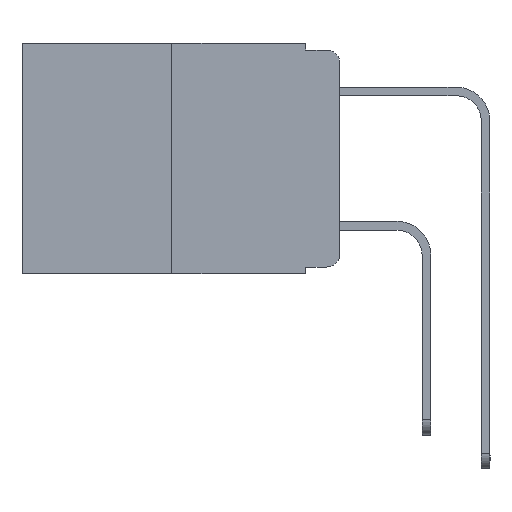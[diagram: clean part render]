
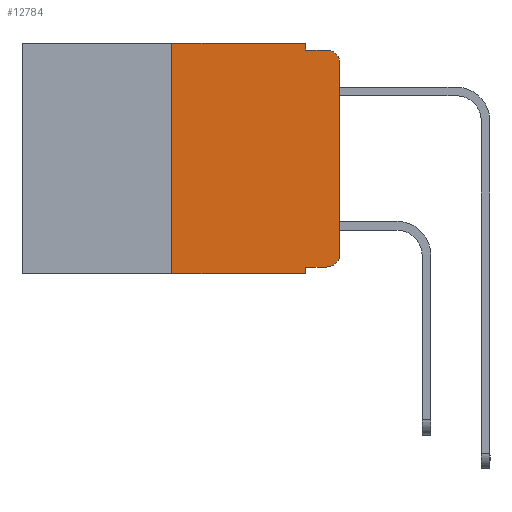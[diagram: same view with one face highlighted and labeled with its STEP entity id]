
A CAD part, left-side view. The second image highlights one B-rep face of the part: STEP entity #12784.
In plain terms, the highlighted planar face has unit normal (-1, 0, 0).
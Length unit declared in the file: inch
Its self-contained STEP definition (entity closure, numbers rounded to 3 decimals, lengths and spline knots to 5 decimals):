
#77 = CARTESIAN_POINT ( 'NONE',  ( 0., 0.051, 0. ) ) ;
#140 = DIRECTION ( 'NONE',  ( 0., 0., -1. ) ) ;
#180 = DIRECTION ( 'NONE',  ( 0., 0., 1. ) ) ;
#378 = VECTOR ( 'NONE', #5971, 39.37008 ) ;
#610 = CARTESIAN_POINT ( 'NONE',  ( 0., 0.051, -0.01 ) ) ;
#616 = LINE ( 'NONE', #4800, #12299 ) ;
#624 = DIRECTION ( 'NONE',  ( 0., -1., 0. ) ) ;
#729 = VERTEX_POINT ( 'NONE', #12332 ) ;
#802 = VECTOR ( 'NONE', #822, 39.37008 ) ;
#822 = DIRECTION ( 'NONE',  ( 0., -1., 0. ) ) ;
#1186 = ORIENTED_EDGE ( 'NONE', *, *, #3852, .T. ) ;
#1196 = ORIENTED_EDGE ( 'NONE', *, *, #6794, .F. ) ;
#1293 = FACE_OUTER_BOUND ( 'NONE', #4846, .T. ) ;
#1451 = ORIENTED_EDGE ( 'NONE', *, *, #1779, .F. ) ;
#1779 = EDGE_CURVE ( 'NONE', #729, #6059, #11518, .T. ) ;
#1817 = ORIENTED_EDGE ( 'NONE', *, *, #9703, .F. ) ;
#1902 = EDGE_CURVE ( 'NONE', #5700, #4947, #2800, .T. ) ;
#2146 = LINE ( 'NONE', #12782, #4140 ) ;
#2340 = DIRECTION ( 'NONE',  ( 0., 0., 1. ) ) ;
#2369 = ORIENTED_EDGE ( 'NONE', *, *, #7929, .T. ) ;
#2800 = CIRCLE ( 'NONE', #13323, 0.02 ) ;
#2854 = CARTESIAN_POINT ( 'NONE',  ( 0., 0.02, -0.333 ) ) ;
#2870 = LINE ( 'NONE', #9394, #802 ) ;
#3072 = CARTESIAN_POINT ( 'NONE',  ( 0., 0.25, -0.343 ) ) ;
#3339 = DIRECTION ( 'NONE',  ( 1., 0., 0. ) ) ;
#3549 = CARTESIAN_POINT ( 'NONE',  ( 0., 0.473, 0. ) ) ;
#3610 = VERTEX_POINT ( 'NONE', #5218 ) ;
#3654 = VECTOR ( 'NONE', #8582, 39.37008 ) ;
#3680 = CARTESIAN_POINT ( 'NONE',  ( 0., 0.051, -0.01 ) ) ;
#3817 = LINE ( 'NONE', #3680, #378 ) ;
#3852 = EDGE_CURVE ( 'NONE', #11744, #11363, #11862, .T. ) ;
#3890 = EDGE_CURVE ( 'NONE', #12164, #11363, #616, .T. ) ;
#4140 = VECTOR ( 'NONE', #2340, 39.37008 ) ;
#4532 = EDGE_CURVE ( 'NONE', #11744, #13049, #2146, .T. ) ;
#4800 = CARTESIAN_POINT ( 'NONE',  ( 0., 0.051, 0. ) ) ;
#4807 = CARTESIAN_POINT ( 'NONE',  ( 0., 0.02, -0.03 ) ) ;
#4846 = EDGE_LOOP ( 'NONE', ( #7281, #13448, #1817, #1451, #1196, #11756, #1186, #13243, #2369, #10557 ) ) ;
#4947 = VERTEX_POINT ( 'NONE', #11326 ) ;
#5218 = CARTESIAN_POINT ( 'NONE',  ( 0., 0., -0.03 ) ) ;
#5402 = CARTESIAN_POINT ( 'NONE',  ( 0., 0., 0. ) ) ;
#5700 = VERTEX_POINT ( 'NONE', #2854 ) ;
#5971 = DIRECTION ( 'NONE',  ( 0., -1., 0. ) ) ;
#6059 = VERTEX_POINT ( 'NONE', #610 ) ;
#6112 = AXIS2_PLACEMENT_3D ( 'NONE', #4807, #13035, #7919 ) ;
#6231 = CARTESIAN_POINT ( 'NONE',  ( 0., 0.051, -0.333 ) ) ;
#6718 = DIRECTION ( 'NONE',  ( -1., 0., 0. ) ) ;
#6727 = CARTESIAN_POINT ( 'NONE',  ( 0., 0.473, -0.343 ) ) ;
#6794 = EDGE_CURVE ( 'NONE', #13049, #729, #2870, .T. ) ;
#6804 = LINE ( 'NONE', #10985, #8304 ) ;
#6867 = DIRECTION ( 'NONE',  ( 0., 0., -1. ) ) ;
#7281 = ORIENTED_EDGE ( 'NONE', *, *, #10033, .T. ) ;
#7380 = VERTEX_POINT ( 'NONE', #11757 ) ;
#7833 = CARTESIAN_POINT ( 'NONE',  ( 0., 0.02, -0.313 ) ) ;
#7866 = CIRCLE ( 'NONE', #6112, 0.02 ) ;
#7919 = DIRECTION ( 'NONE',  ( 0., 0., -1. ) ) ;
#7929 = EDGE_CURVE ( 'NONE', #12164, #5700, #6804, .T. ) ;
#7941 = EDGE_CURVE ( 'NONE', #3610, #7380, #7866, .T. ) ;
#8304 = VECTOR ( 'NONE', #624, 39.37008 ) ;
#8497 = LINE ( 'NONE', #5402, #11776 ) ;
#8582 = DIRECTION ( 'NONE',  ( 0., 0., -1. ) ) ;
#9394 = CARTESIAN_POINT ( 'NONE',  ( 0., 0.473, 0. ) ) ;
#9446 = AXIS2_PLACEMENT_3D ( 'NONE', #3549, #3339, #140 ) ;
#9470 = CARTESIAN_POINT ( 'NONE',  ( 0., 0.051, -0.343 ) ) ;
#9703 = EDGE_CURVE ( 'NONE', #6059, #7380, #3817, .T. ) ;
#10033 = EDGE_CURVE ( 'NONE', #4947, #3610, #8497, .T. ) ;
#10557 = ORIENTED_EDGE ( 'NONE', *, *, #1902, .T. ) ;
#10908 = DIRECTION ( 'NONE',  ( 0., -1., 0. ) ) ;
#10983 = VECTOR ( 'NONE', #10908, 39.37008 ) ;
#10985 = CARTESIAN_POINT ( 'NONE',  ( 0., 0.051, -0.333 ) ) ;
#11326 = CARTESIAN_POINT ( 'NONE',  ( 0., 0., -0.313 ) ) ;
#11363 = VERTEX_POINT ( 'NONE', #9470 ) ;
#11380 = CARTESIAN_POINT ( 'NONE',  ( 0., 0.25, 0. ) ) ;
#11518 = LINE ( 'NONE', #77, #3654 ) ;
#11744 = VERTEX_POINT ( 'NONE', #3072 ) ;
#11756 = ORIENTED_EDGE ( 'NONE', *, *, #4532, .F. ) ;
#11757 = CARTESIAN_POINT ( 'NONE',  ( 0., 0.02, -0.01 ) ) ;
#11776 = VECTOR ( 'NONE', #180, 39.37008 ) ;
#11862 = LINE ( 'NONE', #6727, #10983 ) ;
#11926 = PLANE ( 'NONE',  #9446 ) ;
#12057 = DIRECTION ( 'NONE',  ( 0., 0., -1. ) ) ;
#12164 = VERTEX_POINT ( 'NONE', #6231 ) ;
#12299 = VECTOR ( 'NONE', #6867, 39.37008 ) ;
#12332 = CARTESIAN_POINT ( 'NONE',  ( 0., 0.051, 0. ) ) ;
#12782 = CARTESIAN_POINT ( 'NONE',  ( 0., 0.25, 0. ) ) ;
#12784 = ADVANCED_FACE ( 'NONE', ( #1293 ), #11926, .F. ) ;
#13035 = DIRECTION ( 'NONE',  ( -1., 0., 0. ) ) ;
#13049 = VERTEX_POINT ( 'NONE', #11380 ) ;
#13243 = ORIENTED_EDGE ( 'NONE', *, *, #3890, .F. ) ;
#13323 = AXIS2_PLACEMENT_3D ( 'NONE', #7833, #6718, #12057 ) ;
#13448 = ORIENTED_EDGE ( 'NONE', *, *, #7941, .T. ) ;
